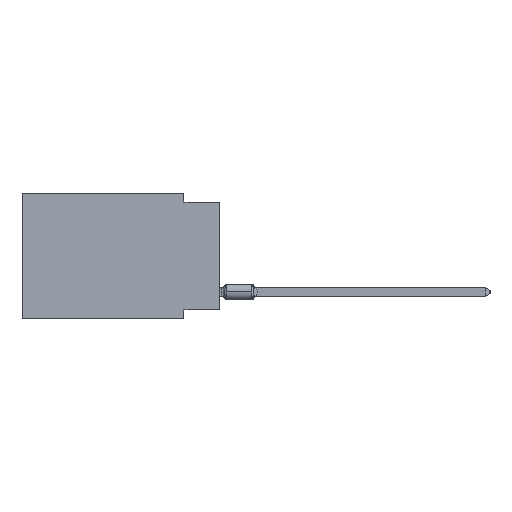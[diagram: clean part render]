
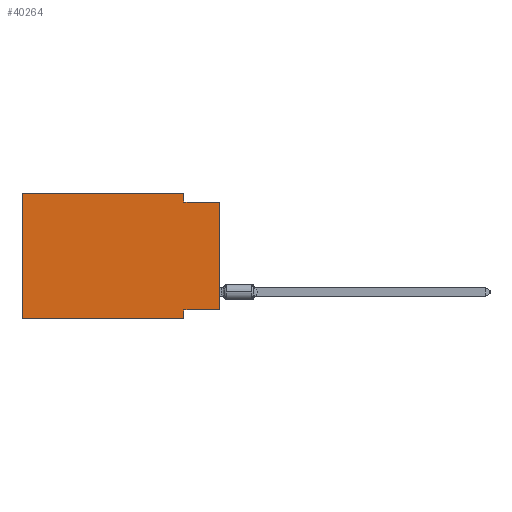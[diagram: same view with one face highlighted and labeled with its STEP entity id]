
A CAD part, left-side view. The second image highlights one B-rep face of the part: STEP entity #40264.
In plain terms, the highlighted planar face has unit normal (-1, 0, 0).
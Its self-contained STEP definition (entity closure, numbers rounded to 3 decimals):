
#9 = CARTESIAN_POINT ( 'NONE',  ( 0., 13.97, 0. ) ) ;
#172 = CARTESIAN_POINT ( 'NONE',  ( 0., 0., 0. ) ) ;
#419 = LINE ( 'NONE', #42593, #6745 ) ;
#493 = ORIENTED_EDGE ( 'NONE', *, *, #10316, .T. ) ;
#664 = VERTEX_POINT ( 'NONE', #22745 ) ;
#2269 = VECTOR ( 'NONE', #29673, 1000. ) ;
#3409 = CARTESIAN_POINT ( 'NONE',  ( 0., 13.97, -8.89 ) ) ;
#3752 = EDGE_CURVE ( 'NONE', #14018, #4060, #36940, .T. ) ;
#4060 = VERTEX_POINT ( 'NONE', #24835 ) ;
#5310 = VECTOR ( 'NONE', #41427, 1000. ) ;
#5520 = DIRECTION ( 'NONE',  ( 0., 1., 0. ) ) ;
#6603 = CARTESIAN_POINT ( 'NONE',  ( 0., 0., -0.635 ) ) ;
#6745 = VECTOR ( 'NONE', #14312, 1000. ) ;
#8831 = AXIS2_PLACEMENT_3D ( 'NONE', #9, #10240, #16431 ) ;
#8952 = CARTESIAN_POINT ( 'NONE',  ( 0., 13.97, 0. ) ) ;
#9941 = CARTESIAN_POINT ( 'NONE',  ( 0., 13.97, 0. ) ) ;
#9954 = VERTEX_POINT ( 'NONE', #30380 ) ;
#10240 = DIRECTION ( 'NONE',  ( 1., 0., 0. ) ) ;
#10316 = EDGE_CURVE ( 'NONE', #16627, #25450, #44921, .T. ) ;
#12237 = CARTESIAN_POINT ( 'NONE',  ( 0., 2.54, -8.89 ) ) ;
#12419 = ORIENTED_EDGE ( 'NONE', *, *, #26399, .F. ) ;
#14018 = VERTEX_POINT ( 'NONE', #28997 ) ;
#14312 = DIRECTION ( 'NONE',  ( 0., 0., -1. ) ) ;
#16005 = CARTESIAN_POINT ( 'NONE',  ( 0., 0., -8.255 ) ) ;
#16431 = DIRECTION ( 'NONE',  ( 0., 0., -1. ) ) ;
#16623 = ORIENTED_EDGE ( 'NONE', *, *, #32771, .F. ) ;
#16627 = VERTEX_POINT ( 'NONE', #36796 ) ;
#17326 = FACE_OUTER_BOUND ( 'NONE', #28352, .T. ) ;
#17330 = DIRECTION ( 'NONE',  ( 0., -1., 0. ) ) ;
#17454 = ORIENTED_EDGE ( 'NONE', *, *, #3752, .F. ) ;
#18793 = LINE ( 'NONE', #8952, #22874 ) ;
#18928 = CARTESIAN_POINT ( 'NONE',  ( 0., 2.54, 0. ) ) ;
#19449 = CARTESIAN_POINT ( 'NONE',  ( 0., 0., -0.635 ) ) ;
#20553 = VERTEX_POINT ( 'NONE', #19449 ) ;
#21738 = VERTEX_POINT ( 'NONE', #22438 ) ;
#21977 = VECTOR ( 'NONE', #31892, 1000. ) ;
#22438 = CARTESIAN_POINT ( 'NONE',  ( 0., 2.54, -8.255 ) ) ;
#22745 = CARTESIAN_POINT ( 'NONE',  ( 0., 13.97, 0. ) ) ;
#22874 = VECTOR ( 'NONE', #36134, 1000. ) ;
#23092 = LINE ( 'NONE', #16005, #31695 ) ;
#24366 = LINE ( 'NONE', #172, #21977 ) ;
#24835 = CARTESIAN_POINT ( 'NONE',  ( 0., 2.54, -0.635 ) ) ;
#25450 = VERTEX_POINT ( 'NONE', #12237 ) ;
#26399 = EDGE_CURVE ( 'NONE', #16627, #664, #31409, .T. ) ;
#27020 = EDGE_CURVE ( 'NONE', #664, #14018, #18793, .T. ) ;
#28053 = ORIENTED_EDGE ( 'NONE', *, *, #44640, .F. ) ;
#28352 = EDGE_LOOP ( 'NONE', ( #36790, #16623, #17454, #34628, #12419, #493, #36085, #28053 ) ) ;
#28997 = CARTESIAN_POINT ( 'NONE',  ( 0., 2.54, 0. ) ) ;
#29673 = DIRECTION ( 'NONE',  ( 0., 0., -1. ) ) ;
#30380 = CARTESIAN_POINT ( 'NONE',  ( 0., 0., -8.255 ) ) ;
#31409 = LINE ( 'NONE', #9941, #5310 ) ;
#31695 = VECTOR ( 'NONE', #5520, 1000. ) ;
#31892 = DIRECTION ( 'NONE',  ( 0., 0., 1. ) ) ;
#32771 = EDGE_CURVE ( 'NONE', #4060, #20553, #44942, .T. ) ;
#34628 = ORIENTED_EDGE ( 'NONE', *, *, #27020, .F. ) ;
#35337 = DIRECTION ( 'NONE',  ( 0., -1., 0. ) ) ;
#36085 = ORIENTED_EDGE ( 'NONE', *, *, #36868, .F. ) ;
#36134 = DIRECTION ( 'NONE',  ( 0., -1., 0. ) ) ;
#36790 = ORIENTED_EDGE ( 'NONE', *, *, #40845, .T. ) ;
#36796 = CARTESIAN_POINT ( 'NONE',  ( 0., 13.97, -8.89 ) ) ;
#36868 = EDGE_CURVE ( 'NONE', #21738, #25450, #419, .T. ) ;
#36940 = LINE ( 'NONE', #18928, #2269 ) ;
#38649 = VECTOR ( 'NONE', #17330, 1000. ) ;
#39707 = VECTOR ( 'NONE', #35337, 1000. ) ;
#40264 = ADVANCED_FACE ( 'NONE', ( #17326 ), #41505, .F. ) ;
#40845 = EDGE_CURVE ( 'NONE', #9954, #20553, #24366, .T. ) ;
#41427 = DIRECTION ( 'NONE',  ( 0., 0., 1. ) ) ;
#41505 = PLANE ( 'NONE',  #8831 ) ;
#42593 = CARTESIAN_POINT ( 'NONE',  ( 0., 2.54, -8.89 ) ) ;
#44640 = EDGE_CURVE ( 'NONE', #9954, #21738, #23092, .T. ) ;
#44921 = LINE ( 'NONE', #3409, #39707 ) ;
#44942 = LINE ( 'NONE', #6603, #38649 ) ;
